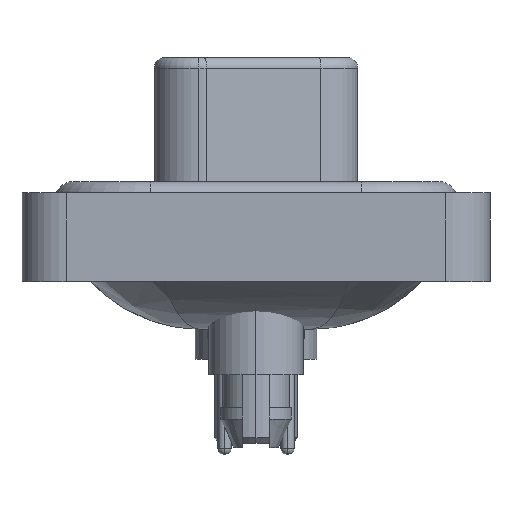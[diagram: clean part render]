
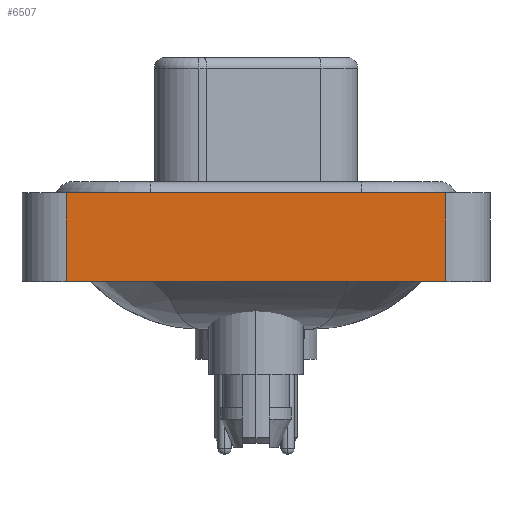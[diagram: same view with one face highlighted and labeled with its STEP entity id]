
A CAD part, left-side view. The second image highlights one B-rep face of the part: STEP entity #6507.
In plain terms, the highlighted planar face has unit normal (-1, 0, 0).
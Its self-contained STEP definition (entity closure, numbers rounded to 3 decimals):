
#722 = CARTESIAN_POINT ( 'NONE',  ( -7.25, -8.55, -3.6 ) ) ;
#1244 = VECTOR ( 'NONE', #1755, 1000. ) ;
#1754 = EDGE_CURVE ( 'NONE', #8896, #16493, #12567, .T. ) ;
#1755 = DIRECTION ( 'NONE',  ( 0., 0., 1. ) ) ;
#2296 = ORIENTED_EDGE ( 'NONE', *, *, #5060, .T. ) ;
#2426 = VERTEX_POINT ( 'NONE', #4470 ) ;
#3881 = DIRECTION ( 'NONE',  ( -1., 0., 0. ) ) ;
#4470 = CARTESIAN_POINT ( 'NONE',  ( -7.25, -8.55, 0.4 ) ) ;
#4576 = VECTOR ( 'NONE', #6407, 1000. ) ;
#4796 = CARTESIAN_POINT ( 'NONE',  ( -7.25, 8.55, 0.4 ) ) ;
#5060 = EDGE_CURVE ( 'NONE', #5210, #2426, #14558, .T. ) ;
#5210 = VERTEX_POINT ( 'NONE', #16781 ) ;
#6127 = EDGE_LOOP ( 'NONE', ( #2296, #7525, #15959, #10829 ) ) ;
#6407 = DIRECTION ( 'NONE',  ( 0., -1., 0. ) ) ;
#6507 = ADVANCED_FACE ( 'NONE', ( #15355 ), #12298, .T. ) ;
#6660 = CARTESIAN_POINT ( 'NONE',  ( -7.25, -8.55, -3.6 ) ) ;
#7223 = EDGE_CURVE ( 'NONE', #8896, #5210, #13525, .T. ) ;
#7525 = ORIENTED_EDGE ( 'NONE', *, *, #13524, .F. ) ;
#8240 = CARTESIAN_POINT ( 'NONE',  ( -7.25, 8.55, -3.6 ) ) ;
#8270 = VECTOR ( 'NONE', #18435, 1000. ) ;
#8431 = DIRECTION ( 'NONE',  ( 0., 0., 1. ) ) ;
#8896 = VERTEX_POINT ( 'NONE', #16663 ) ;
#9275 = LINE ( 'NONE', #10771, #17545 ) ;
#10771 = CARTESIAN_POINT ( 'NONE',  ( -7.25, -8.55, 0.4 ) ) ;
#10829 = ORIENTED_EDGE ( 'NONE', *, *, #7223, .T. ) ;
#11122 = AXIS2_PLACEMENT_3D ( 'NONE', #6660, #3881, #8431 ) ;
#12298 = PLANE ( 'NONE',  #11122 ) ;
#12567 = LINE ( 'NONE', #8240, #8270 ) ;
#13524 = EDGE_CURVE ( 'NONE', #16493, #2426, #9275, .T. ) ;
#13525 = LINE ( 'NONE', #722, #4576 ) ;
#14558 = LINE ( 'NONE', #14649, #1244 ) ;
#14649 = CARTESIAN_POINT ( 'NONE',  ( -7.25, -8.55, -3.6 ) ) ;
#14994 = DIRECTION ( 'NONE',  ( 0., -1., 0. ) ) ;
#15355 = FACE_OUTER_BOUND ( 'NONE', #6127, .T. ) ;
#15959 = ORIENTED_EDGE ( 'NONE', *, *, #1754, .F. ) ;
#16493 = VERTEX_POINT ( 'NONE', #4796 ) ;
#16663 = CARTESIAN_POINT ( 'NONE',  ( -7.25, 8.55, -3.6 ) ) ;
#16781 = CARTESIAN_POINT ( 'NONE',  ( -7.25, -8.55, -3.6 ) ) ;
#17545 = VECTOR ( 'NONE', #14994, 1000. ) ;
#18435 = DIRECTION ( 'NONE',  ( 0., 0., 1. ) ) ;
